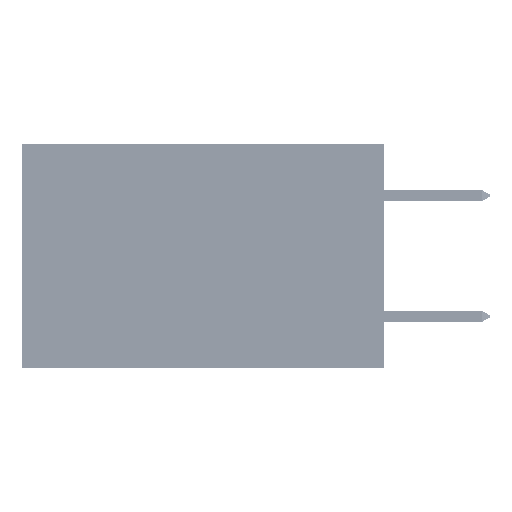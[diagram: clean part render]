
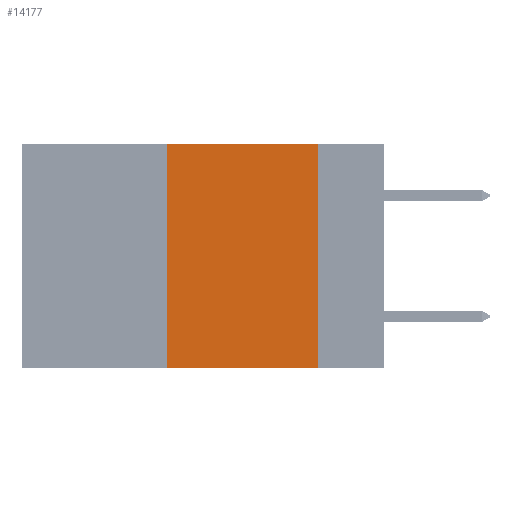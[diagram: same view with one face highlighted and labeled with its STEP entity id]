
A CAD part, left-side view. The second image highlights one B-rep face of the part: STEP entity #14177.
In plain terms, the highlighted planar face has unit normal (-1, 0, 0).
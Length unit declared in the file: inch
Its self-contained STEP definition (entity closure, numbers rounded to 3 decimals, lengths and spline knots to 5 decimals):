
#691 = CARTESIAN_POINT ( 'NONE',  ( 0., 0.6, 0. ) ) ;
#1276 = EDGE_CURVE ( 'NONE', #51083, #21293, #19290, .T. ) ;
#3342 = CARTESIAN_POINT ( 'NONE',  ( 0., 0.6, -0.37 ) ) ;
#3891 = LINE ( 'NONE', #39768, #33004 ) ;
#4993 = LINE ( 'NONE', #29940, #49608 ) ;
#6291 = CARTESIAN_POINT ( 'NONE',  ( 0., 0.11, -0.37 ) ) ;
#8422 = AXIS2_PLACEMENT_3D ( 'NONE', #691, #16395, #28079 ) ;
#9952 = LINE ( 'NONE', #29881, #27518 ) ;
#11309 = DIRECTION ( 'NONE',  ( 0., -1., 0. ) ) ;
#13949 = DIRECTION ( 'NONE',  ( 0., -1., 0. ) ) ;
#14177 = ADVANCED_FACE ( 'NONE', ( #20118 ), #20381, .F. ) ;
#16395 = DIRECTION ( 'NONE',  ( 1., 0., 0. ) ) ;
#19290 = LINE ( 'NONE', #3342, #20257 ) ;
#20118 = FACE_OUTER_BOUND ( 'NONE', #21431, .T. ) ;
#20257 = VECTOR ( 'NONE', #11309, 39.37008 ) ;
#20381 = PLANE ( 'NONE',  #8422 ) ;
#21190 = DIRECTION ( 'NONE',  ( 0., 0., 1. ) ) ;
#21293 = VERTEX_POINT ( 'NONE', #6291 ) ;
#21431 = EDGE_LOOP ( 'NONE', ( #47589, #24534, #42750, #33599 ) ) ;
#21783 = EDGE_CURVE ( 'NONE', #31200, #42402, #9952, .T. ) ;
#24534 = ORIENTED_EDGE ( 'NONE', *, *, #21783, .F. ) ;
#27518 = VECTOR ( 'NONE', #13949, 39.37008 ) ;
#28079 = DIRECTION ( 'NONE',  ( 0., 0., -1. ) ) ;
#29279 = EDGE_CURVE ( 'NONE', #42402, #21293, #3891, .T. ) ;
#29881 = CARTESIAN_POINT ( 'NONE',  ( 0., 0.6, 0. ) ) ;
#29940 = CARTESIAN_POINT ( 'NONE',  ( 0., 0.36, 0. ) ) ;
#31200 = VERTEX_POINT ( 'NONE', #32518 ) ;
#31512 = CARTESIAN_POINT ( 'NONE',  ( 0., 0.36, -0.37 ) ) ;
#32518 = CARTESIAN_POINT ( 'NONE',  ( 0., 0.36, 0. ) ) ;
#33004 = VECTOR ( 'NONE', #47748, 39.37008 ) ;
#33599 = ORIENTED_EDGE ( 'NONE', *, *, #1276, .T. ) ;
#38358 = CARTESIAN_POINT ( 'NONE',  ( 0., 0.11, 0. ) ) ;
#39768 = CARTESIAN_POINT ( 'NONE',  ( 0., 0.11, 0. ) ) ;
#42402 = VERTEX_POINT ( 'NONE', #38358 ) ;
#42750 = ORIENTED_EDGE ( 'NONE', *, *, #43714, .F. ) ;
#43714 = EDGE_CURVE ( 'NONE', #51083, #31200, #4993, .T. ) ;
#47589 = ORIENTED_EDGE ( 'NONE', *, *, #29279, .F. ) ;
#47748 = DIRECTION ( 'NONE',  ( 0., 0., -1. ) ) ;
#49608 = VECTOR ( 'NONE', #21190, 39.37008 ) ;
#51083 = VERTEX_POINT ( 'NONE', #31512 ) ;
